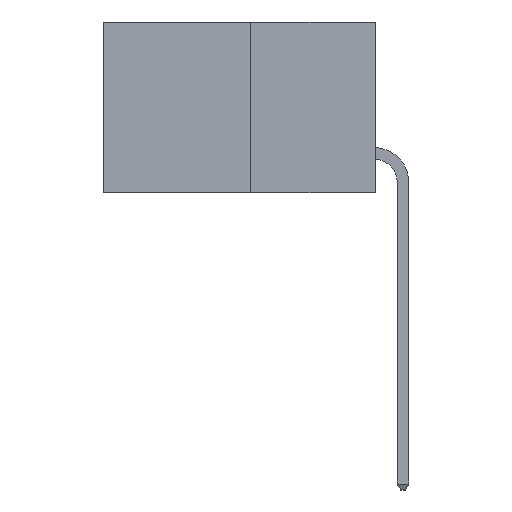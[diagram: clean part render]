
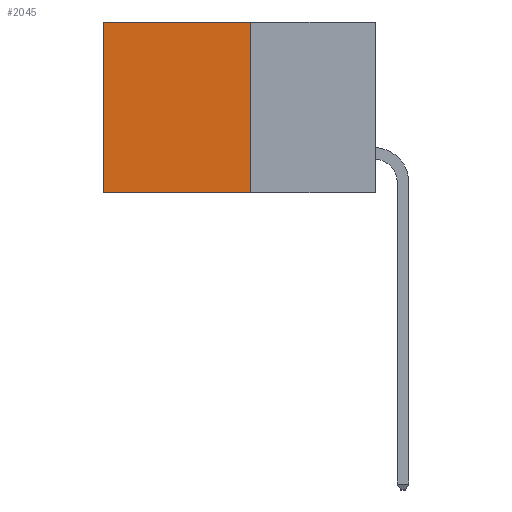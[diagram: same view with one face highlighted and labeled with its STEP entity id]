
A CAD part, left-side view. The second image highlights one B-rep face of the part: STEP entity #2045.
In plain terms, the highlighted planar face has unit normal (-1, 0, 0).
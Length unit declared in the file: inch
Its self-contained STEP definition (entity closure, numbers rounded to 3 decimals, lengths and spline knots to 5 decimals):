
#65 = CARTESIAN_POINT ( 'NONE',  ( 0.277, 0.59, 0. ) ) ;
#81 = CARTESIAN_POINT ( 'NONE',  ( 0.277, 0.27, 0. ) ) ;
#106 = EDGE_CURVE ( 'NONE', #1924, #2996, #6428, .T. ) ;
#371 = CARTESIAN_POINT ( 'NONE',  ( 0.277, 0.27, -0.37 ) ) ;
#475 = ORIENTED_EDGE ( 'NONE', *, *, #106, .F. ) ;
#1636 = CARTESIAN_POINT ( 'NONE',  ( 0.277, 0.59, -0.37 ) ) ;
#1924 = VERTEX_POINT ( 'NONE', #81 ) ;
#2045 = ADVANCED_FACE ( 'NONE', ( #8055 ), #7536, .F. ) ;
#2393 = DIRECTION ( 'NONE',  ( 0., 0., -1. ) ) ;
#2823 = EDGE_CURVE ( 'NONE', #1924, #6343, #9124, .T. ) ;
#2996 = VERTEX_POINT ( 'NONE', #7129 ) ;
#3791 = DIRECTION ( 'NONE',  ( 0., 0., -1. ) ) ;
#4031 = EDGE_LOOP ( 'NONE', ( #5211, #4428, #475, #4143 ) ) ;
#4115 = CARTESIAN_POINT ( 'NONE',  ( 0.277, 0.59, -0.37 ) ) ;
#4143 = ORIENTED_EDGE ( 'NONE', *, *, #2823, .T. ) ;
#4428 = ORIENTED_EDGE ( 'NONE', *, *, #5416, .F. ) ;
#4503 = VECTOR ( 'NONE', #3791, 39.37008 ) ;
#4556 = CARTESIAN_POINT ( 'NONE',  ( 0.277, 0.27, -0.37 ) ) ;
#5211 = ORIENTED_EDGE ( 'NONE', *, *, #6324, .T. ) ;
#5292 = VERTEX_POINT ( 'NONE', #4115 ) ;
#5416 = EDGE_CURVE ( 'NONE', #2996, #5292, #6335, .T. ) ;
#5533 = AXIS2_PLACEMENT_3D ( 'NONE', #371, #7554, #7651 ) ;
#6106 = VECTOR ( 'NONE', #7089, 39.37008 ) ;
#6324 = EDGE_CURVE ( 'NONE', #6343, #5292, #8780, .T. ) ;
#6335 = LINE ( 'NONE', #8477, #6106 ) ;
#6343 = VERTEX_POINT ( 'NONE', #65 ) ;
#6428 = LINE ( 'NONE', #4556, #4503 ) ;
#7089 = DIRECTION ( 'NONE',  ( 0., 1., 0. ) ) ;
#7129 = CARTESIAN_POINT ( 'NONE',  ( 0.277, 0.27, -0.37 ) ) ;
#7477 = VECTOR ( 'NONE', #9250, 39.37008 ) ;
#7536 = PLANE ( 'NONE',  #5533 ) ;
#7554 = DIRECTION ( 'NONE',  ( 1., 0., 0. ) ) ;
#7651 = DIRECTION ( 'NONE',  ( 0., 0., -1. ) ) ;
#8055 = FACE_OUTER_BOUND ( 'NONE', #4031, .T. ) ;
#8477 = CARTESIAN_POINT ( 'NONE',  ( 0.277, 0.27, -0.37 ) ) ;
#8780 = LINE ( 'NONE', #1636, #8999 ) ;
#8999 = VECTOR ( 'NONE', #2393, 39.37008 ) ;
#9124 = LINE ( 'NONE', #9277, #7477 ) ;
#9250 = DIRECTION ( 'NONE',  ( 0., 1., 0. ) ) ;
#9277 = CARTESIAN_POINT ( 'NONE',  ( 0.277, 0.27, 0. ) ) ;
